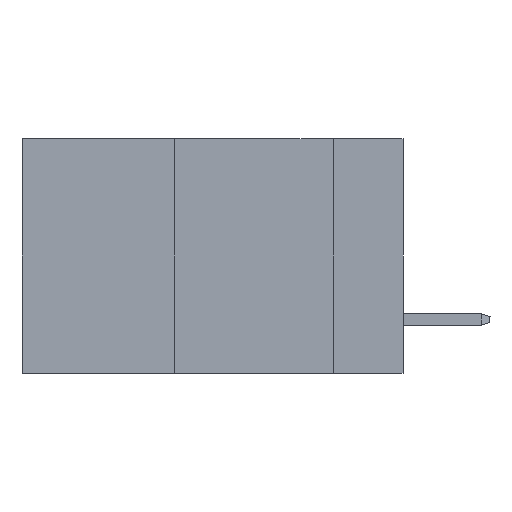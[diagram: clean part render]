
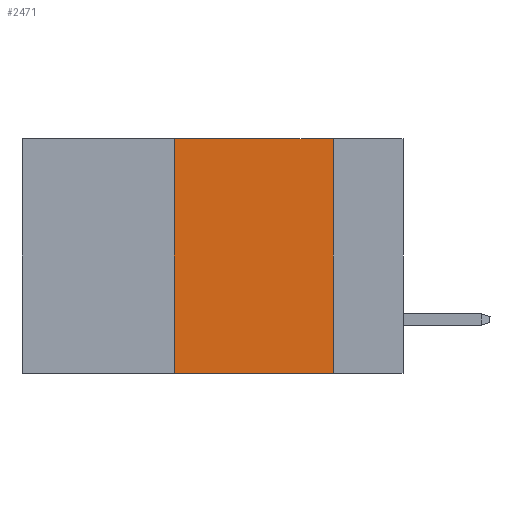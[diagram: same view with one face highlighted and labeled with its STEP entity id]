
A CAD part, left-side view. The second image highlights one B-rep face of the part: STEP entity #2471.
In plain terms, the highlighted planar face has unit normal (-1, 0, 0).
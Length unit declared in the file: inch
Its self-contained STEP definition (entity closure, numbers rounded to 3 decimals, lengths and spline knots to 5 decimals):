
#354 = VECTOR ( 'NONE', #7725, 39.37008 ) ;
#758 = CARTESIAN_POINT ( 'NONE',  ( 0., 0.11, 0. ) ) ;
#1283 = CARTESIAN_POINT ( 'NONE',  ( 0., 0.11, 0. ) ) ;
#2000 = VECTOR ( 'NONE', #15122, 39.37008 ) ;
#2471 = ADVANCED_FACE ( 'NONE', ( #26563 ), #10272, .F. ) ;
#4147 = VERTEX_POINT ( 'NONE', #758 ) ;
#4249 = VERTEX_POINT ( 'NONE', #10222 ) ;
#5078 = EDGE_LOOP ( 'NONE', ( #24374, #24894, #12925, #6210 ) ) ;
#6210 = ORIENTED_EDGE ( 'NONE', *, *, #22422, .T. ) ;
#6847 = CARTESIAN_POINT ( 'NONE',  ( 0., 0.6, -0.37 ) ) ;
#7725 = DIRECTION ( 'NONE',  ( 0., -1., 0. ) ) ;
#8876 = LINE ( 'NONE', #6847, #2000 ) ;
#8957 = EDGE_CURVE ( 'NONE', #15545, #4147, #12047, .T. ) ;
#9636 = CARTESIAN_POINT ( 'NONE',  ( 0., 0.6, 0. ) ) ;
#9854 = LINE ( 'NONE', #1283, #16927 ) ;
#10129 = CARTESIAN_POINT ( 'NONE',  ( 0., 0.6, 0. ) ) ;
#10222 = CARTESIAN_POINT ( 'NONE',  ( 0., 0.36, -0.37 ) ) ;
#10272 = PLANE ( 'NONE',  #21625 ) ;
#12047 = LINE ( 'NONE', #9636, #354 ) ;
#12925 = ORIENTED_EDGE ( 'NONE', *, *, #26174, .F. ) ;
#13776 = EDGE_CURVE ( 'NONE', #4147, #18558, #9854, .T. ) ;
#13863 = CARTESIAN_POINT ( 'NONE',  ( 0., 0.36, 0. ) ) ;
#13997 = DIRECTION ( 'NONE',  ( 0., 0., 1. ) ) ;
#15122 = DIRECTION ( 'NONE',  ( 0., -1., 0. ) ) ;
#15545 = VERTEX_POINT ( 'NONE', #23477 ) ;
#15956 = DIRECTION ( 'NONE',  ( 0., 0., -1. ) ) ;
#16227 = DIRECTION ( 'NONE',  ( 1., 0., 0. ) ) ;
#16927 = VECTOR ( 'NONE', #15956, 39.37008 ) ;
#18558 = VERTEX_POINT ( 'NONE', #21144 ) ;
#21144 = CARTESIAN_POINT ( 'NONE',  ( 0., 0.11, -0.37 ) ) ;
#21625 = AXIS2_PLACEMENT_3D ( 'NONE', #10129, #16227, #24648 ) ;
#22422 = EDGE_CURVE ( 'NONE', #4249, #18558, #8876, .T. ) ;
#23267 = VECTOR ( 'NONE', #13997, 39.37008 ) ;
#23477 = CARTESIAN_POINT ( 'NONE',  ( 0., 0.36, 0. ) ) ;
#23928 = LINE ( 'NONE', #13863, #23267 ) ;
#24374 = ORIENTED_EDGE ( 'NONE', *, *, #13776, .F. ) ;
#24648 = DIRECTION ( 'NONE',  ( 0., 0., -1. ) ) ;
#24894 = ORIENTED_EDGE ( 'NONE', *, *, #8957, .F. ) ;
#26174 = EDGE_CURVE ( 'NONE', #4249, #15545, #23928, .T. ) ;
#26563 = FACE_OUTER_BOUND ( 'NONE', #5078, .T. ) ;
